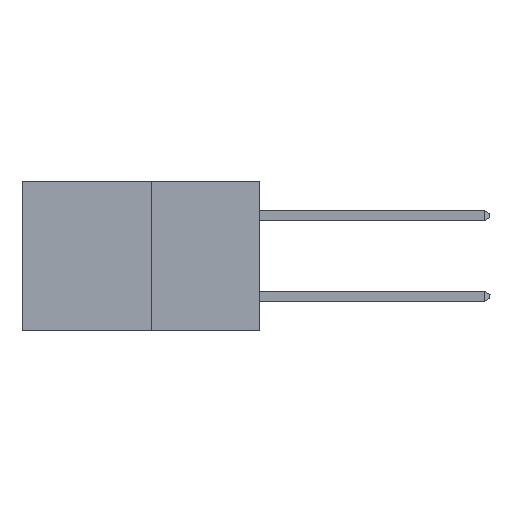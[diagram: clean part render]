
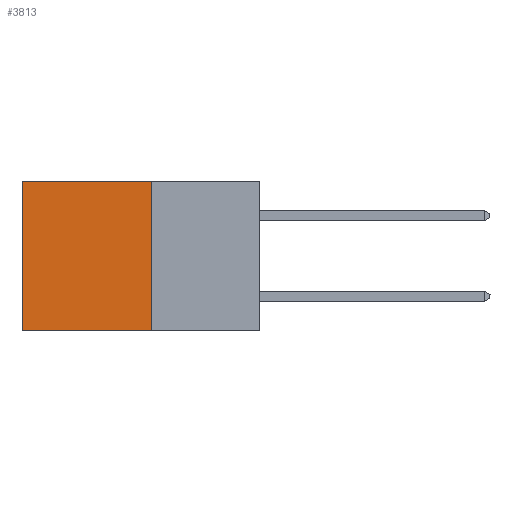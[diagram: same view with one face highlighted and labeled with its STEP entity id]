
A CAD part, left-side view. The second image highlights one B-rep face of the part: STEP entity #3813.
In plain terms, the highlighted planar face has unit normal (-1, 0, 0).
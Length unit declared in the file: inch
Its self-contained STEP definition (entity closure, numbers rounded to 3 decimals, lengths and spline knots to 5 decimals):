
#575 = EDGE_LOOP ( 'NONE', ( #17073, #24732, #19957, #4199 ) ) ;
#646 = LINE ( 'NONE', #9783, #13183 ) ;
#1139 = VERTEX_POINT ( 'NONE', #20688 ) ;
#2503 = LINE ( 'NONE', #15294, #23699 ) ;
#3813 = ADVANCED_FACE ( 'NONE', ( #25760 ), #15237, .F. ) ;
#3900 = VERTEX_POINT ( 'NONE', #21080 ) ;
#4199 = ORIENTED_EDGE ( 'NONE', *, *, #12776, .T. ) ;
#4754 = DIRECTION ( 'NONE',  ( 0., 1., 0. ) ) ;
#6383 = VERTEX_POINT ( 'NONE', #20717 ) ;
#7344 = CARTESIAN_POINT ( 'NONE',  ( 0.277, 0.27, -0.37 ) ) ;
#8907 = AXIS2_PLACEMENT_3D ( 'NONE', #23002, #23436, #17009 ) ;
#9783 = CARTESIAN_POINT ( 'NONE',  ( 0.277, 0.27, 0. ) ) ;
#11719 = EDGE_CURVE ( 'NONE', #3900, #1139, #2503, .T. ) ;
#12169 = VECTOR ( 'NONE', #17684, 39.37008 ) ;
#12776 = EDGE_CURVE ( 'NONE', #6383, #3900, #646, .T. ) ;
#13183 = VECTOR ( 'NONE', #20107, 39.37008 ) ;
#14568 = VERTEX_POINT ( 'NONE', #15192 ) ;
#15192 = CARTESIAN_POINT ( 'NONE',  ( 0.277, 0.27, -0.37 ) ) ;
#15237 = PLANE ( 'NONE',  #8907 ) ;
#15294 = CARTESIAN_POINT ( 'NONE',  ( 0.277, 0.59, -0.37 ) ) ;
#15478 = VECTOR ( 'NONE', #4754, 39.37008 ) ;
#17009 = DIRECTION ( 'NONE',  ( 0., 0., -1. ) ) ;
#17073 = ORIENTED_EDGE ( 'NONE', *, *, #11719, .T. ) ;
#17331 = DIRECTION ( 'NONE',  ( 0., 0., -1. ) ) ;
#17684 = DIRECTION ( 'NONE',  ( 0., 0., -1. ) ) ;
#19957 = ORIENTED_EDGE ( 'NONE', *, *, #22615, .F. ) ;
#20107 = DIRECTION ( 'NONE',  ( 0., 1., 0. ) ) ;
#20472 = EDGE_CURVE ( 'NONE', #14568, #1139, #26340, .T. ) ;
#20688 = CARTESIAN_POINT ( 'NONE',  ( 0.277, 0.59, -0.37 ) ) ;
#20717 = CARTESIAN_POINT ( 'NONE',  ( 0.277, 0.27, 0. ) ) ;
#21080 = CARTESIAN_POINT ( 'NONE',  ( 0.277, 0.59, 0. ) ) ;
#21189 = CARTESIAN_POINT ( 'NONE',  ( 0.277, 0.27, -0.37 ) ) ;
#22615 = EDGE_CURVE ( 'NONE', #6383, #14568, #23054, .T. ) ;
#23002 = CARTESIAN_POINT ( 'NONE',  ( 0.277, 0.27, -0.37 ) ) ;
#23054 = LINE ( 'NONE', #7344, #12169 ) ;
#23436 = DIRECTION ( 'NONE',  ( 1., 0., 0. ) ) ;
#23699 = VECTOR ( 'NONE', #17331, 39.37008 ) ;
#24732 = ORIENTED_EDGE ( 'NONE', *, *, #20472, .F. ) ;
#25760 = FACE_OUTER_BOUND ( 'NONE', #575, .T. ) ;
#26340 = LINE ( 'NONE', #21189, #15478 ) ;
